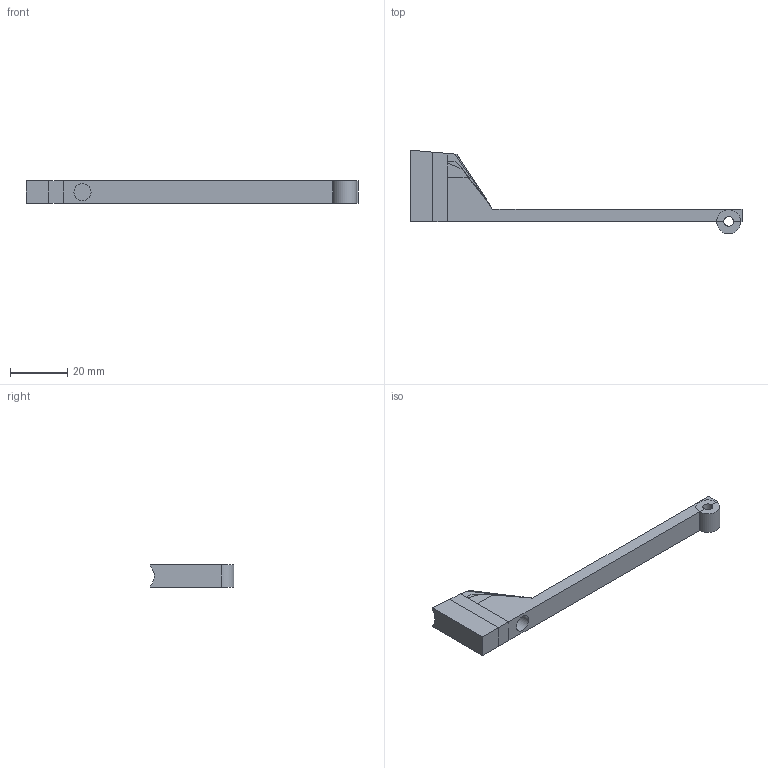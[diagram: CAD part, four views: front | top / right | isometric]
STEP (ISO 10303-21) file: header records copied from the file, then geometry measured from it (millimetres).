
FILE_DESCRIPTION(('FreeCAD Model'),'2;1');
FILE_NAME('ejector arm.step', '2015-07-10T13:15:53',('Author'),(''), 'Open CASCADE STEP processor 6.8','FreeCAD','Unknown');
FILE_SCHEMA(('AUTOMOTIVE_DESIGN_CC2 { 1 2 10303 214 -1 1 5 4 }'));
Length unit declared in the file: millimetre
Products named in the file (1): Pocket006
Bounding box: 116 x 29.21 x 8 mm (x, y, z)
Volume: 7459.1 mm3; surface area: 4401.9 mm2
Topology: 1 solids, 1 shells, 46 faces, 118 edges, 73 vertices
Faces by surface type: plane 39, cylinder 7
Full cylindrical faces by diameter (mm): 6 x1
Entity records: 2961 total; most frequent: CARTESIAN_POINT 626, DIRECTION 416, LINE 284, VECTOR 284, ORIENTED_EDGE 236, PCURVE 236, DEFINITIONAL_REPRESENTATION 236, EDGE_CURVE 118
